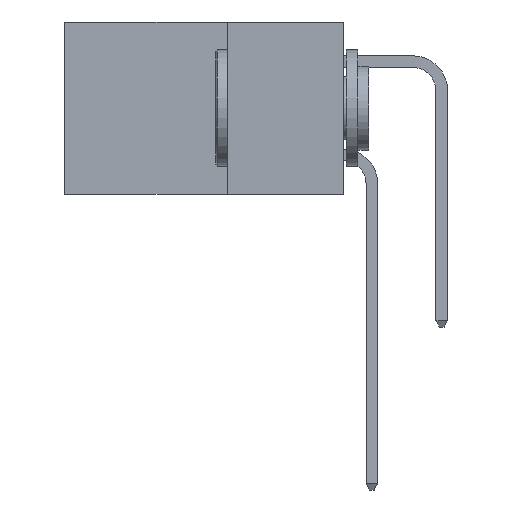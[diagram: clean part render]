
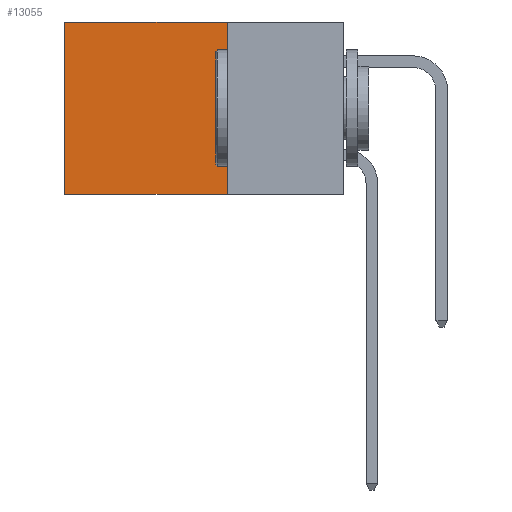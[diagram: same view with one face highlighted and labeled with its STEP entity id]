
A CAD part, left-side view. The second image highlights one B-rep face of the part: STEP entity #13055.
In plain terms, the highlighted planar face has unit normal (-1, 0, 0).
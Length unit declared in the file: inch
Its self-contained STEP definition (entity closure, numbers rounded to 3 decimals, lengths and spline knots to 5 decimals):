
#38 = ORIENTED_EDGE ( 'NONE', *, *, #14770, .T. ) ;
#41 = ORIENTED_EDGE ( 'NONE', *, *, #9154, .F. ) ;
#74 = ORIENTED_EDGE ( 'NONE', *, *, #14418, .F. ) ;
#125 = ORIENTED_EDGE ( 'NONE', *, *, #12025, .T. ) ;
#396 = CARTESIAN_POINT ( 'NONE',  ( 0.2615, 0.6, 0. ) ) ;
#654 = CARTESIAN_POINT ( 'NONE',  ( 0.2615, 0.25, 0. ) ) ;
#1061 = DIRECTION ( 'NONE',  ( 0., 0., -1. ) ) ;
#1261 = VECTOR ( 'NONE', #3803, 39.37008 ) ;
#1751 = CARTESIAN_POINT ( 'NONE',  ( 0.2615, 0.6, -0.37 ) ) ;
#2671 = FACE_OUTER_BOUND ( 'NONE', #4937, .T. ) ;
#3803 = DIRECTION ( 'NONE',  ( 0., 1., 0. ) ) ;
#4713 = CARTESIAN_POINT ( 'NONE',  ( 0.2615, 0.25, -0.37 ) ) ;
#4937 = EDGE_LOOP ( 'NONE', ( #38, #41, #74, #125 ) ) ;
#4959 = LINE ( 'NONE', #12812, #10845 ) ;
#5085 = CARTESIAN_POINT ( 'NONE',  ( 0.2615, 0.25, -0.37 ) ) ;
#5375 = DIRECTION ( 'NONE',  ( 0., 0., -1. ) ) ;
#5416 = VECTOR ( 'NONE', #5375, 39.37008 ) ;
#5522 = VERTEX_POINT ( 'NONE', #10610 ) ;
#5561 = VERTEX_POINT ( 'NONE', #7778 ) ;
#5687 = DIRECTION ( 'NONE',  ( 0., 0., -1. ) ) ;
#5701 = DIRECTION ( 'NONE',  ( 1., 0., 0. ) ) ;
#5719 = PLANE ( 'NONE',  #6729 ) ;
#5803 = CARTESIAN_POINT ( 'NONE',  ( 0.2615, 0.25, -0.37 ) ) ;
#6729 = AXIS2_PLACEMENT_3D ( 'NONE', #5803, #5701, #5687 ) ;
#7619 = VERTEX_POINT ( 'NONE', #654 ) ;
#7778 = CARTESIAN_POINT ( 'NONE',  ( 0.2615, 0.6, -0.37 ) ) ;
#8600 = LINE ( 'NONE', #1751, #5416 ) ;
#8645 = VERTEX_POINT ( 'NONE', #396 ) ;
#9154 = EDGE_CURVE ( 'NONE', #5522, #5561, #10405, .T. ) ;
#10405 = LINE ( 'NONE', #5085, #1261 ) ;
#10610 = CARTESIAN_POINT ( 'NONE',  ( 0.2615, 0.25, -0.37 ) ) ;
#10845 = VECTOR ( 'NONE', #12781, 39.37008 ) ;
#10953 = VECTOR ( 'NONE', #1061, 39.37008 ) ;
#11322 = LINE ( 'NONE', #4713, #10953 ) ;
#12025 = EDGE_CURVE ( 'NONE', #7619, #8645, #4959, .T. ) ;
#12781 = DIRECTION ( 'NONE',  ( 0., 1., 0. ) ) ;
#12812 = CARTESIAN_POINT ( 'NONE',  ( 0.2615, 0.25, 0. ) ) ;
#13055 = ADVANCED_FACE ( 'NONE', ( #2671 ), #5719, .F. ) ;
#14418 = EDGE_CURVE ( 'NONE', #7619, #5522, #11322, .T. ) ;
#14770 = EDGE_CURVE ( 'NONE', #8645, #5561, #8600, .T. ) ;
